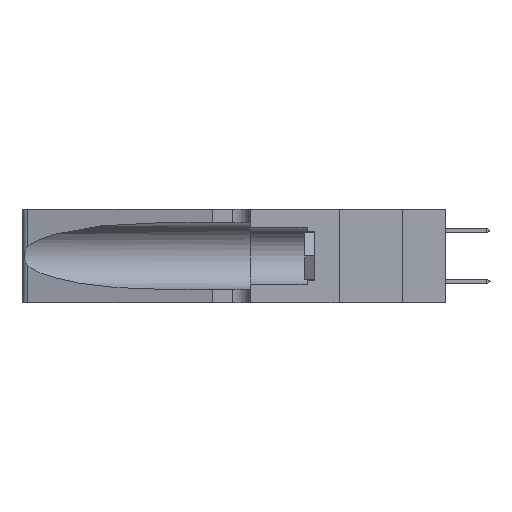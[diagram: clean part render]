
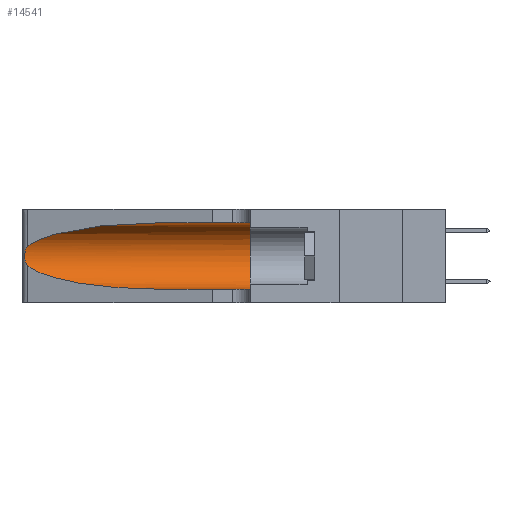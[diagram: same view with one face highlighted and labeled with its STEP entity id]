
A CAD part, left-side view. The second image highlights one B-rep face of the part: STEP entity #14541.
In plain terms, the highlighted cylindrical face has radius 3.308 mm (diameter 6.617 mm), a partial arc.
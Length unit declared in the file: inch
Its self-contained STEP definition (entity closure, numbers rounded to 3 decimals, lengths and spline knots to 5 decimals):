
#385 = ORIENTED_EDGE ( 'NONE', *, *, #40518, .T. ) ;
#543 = VERTEX_POINT ( 'NONE', #14534 ) ;
#595 = VERTEX_POINT ( 'NONE', #36358 ) ;
#2200 = CARTESIAN_POINT ( 'NONE',  ( 0.25639, 1.23186, 0.15144 ) ) ;
#2887 = CARTESIAN_POINT ( 'NONE',  ( 0.1305, 0.35, 0.31525 ) ) ;
#3528 = CARTESIAN_POINT ( 'NONE',  ( 0.25854, 1.2359, 0.20912 ) ) ;
#3661 = CARTESIAN_POINT ( 'NONE',  ( 0.25639, 1.23184, 0.21858 ) ) ;
#4517 = VECTOR ( 'NONE', #16160, 39.37008 ) ;
#4999 = DIRECTION ( 'NONE',  ( 0., -1., 0. ) ) ;
#6022 = VERTEX_POINT ( 'NONE', #2887 ) ;
#6552 = DIRECTION ( 'NONE',  ( 0., 0., 1. ) ) ;
#7584 = EDGE_CURVE ( 'NONE', #6022, #31005, #39950, .T. ) ;
#8187 = CARTESIAN_POINT ( 'NONE',  ( 0.26075, 1.23896, 0.178 ) ) ;
#11516 = LINE ( 'NONE', #19167, #4517 ) ;
#11859 = B_SPLINE_CURVE_WITH_KNOTS ( 'NONE', 3,
 ( #23748, #30055, #3661, #22362, #3528, #25611, #33675, #8187, #33401, #37580, #30331, #2200, #39976, #13443 ),
 .UNSPECIFIED., .F., .F.,
 ( 4, 2, 2, 2, 2, 2, 4 ),
 ( 0., 0.00027, 0.00053, 0.00107, 0.0016, 0.00187, 0.00214 ),
 .UNSPECIFIED. ) ;
#12293 = AXIS2_PLACEMENT_3D ( 'NONE', #34263, #28119, #6552 ) ;
#12368 = FACE_OUTER_BOUND ( 'NONE', #39198, .T. ) ;
#12741 = EDGE_CURVE ( 'NONE', #38311, #595, #11859, .T. ) ;
#13443 = CARTESIAN_POINT ( 'NONE',  ( 0.25487, 1.22718, 0.14631 ) ) ;
#14308 = ORIENTED_EDGE ( 'NONE', *, *, #7584, .F. ) ;
#14534 = CARTESIAN_POINT ( 'NONE',  ( 0.1305, 0.72297, 0.31525 ) ) ;
#14541 = ADVANCED_FACE ( 'NONE', ( #12368 ), #28504, .F. ) ;
#15064 = AXIS2_PLACEMENT_3D ( 'NONE', #24223, #4999, #30131 ) ;
#15164 = EDGE_CURVE ( 'NONE', #543, #6022, #23101, .T. ) ;
#15820 = CARTESIAN_POINT ( 'NONE',  ( 0.25487, 1.22718, 0.22369 ) ) ;
#16160 = DIRECTION ( 'NONE',  ( 0., -1., 0. ) ) ;
#17326 = CARTESIAN_POINT ( 'NONE',  ( 0.18966, 0.96281, 0.05475 ) ) ;
#19167 = CARTESIAN_POINT ( 'NONE',  ( 0.1305, 1.61858, 0.05475 ) ) ;
#19524 = CARTESIAN_POINT ( 'NONE',  ( 0.18966, 0.96281, 0.31525 ) ) ;
#19714 = VECTOR ( 'NONE', #20458, 39.37008 ) ;
#20053 = CARTESIAN_POINT ( 'NONE',  ( 0.1305, 0.72297, 0.05475 ) ) ;
#20215 = ORIENTED_EDGE ( 'NONE', *, *, #15164, .F. ) ;
#20458 = DIRECTION ( 'NONE',  ( 0., -1., 0. ) ) ;
#21467 = CARTESIAN_POINT ( 'NONE',  ( 0.1305, 0.72297, 0.31525 ) ) ;
#21906 = EDGE_CURVE ( 'NONE', #543, #38311, #23351, .T. ) ;
#22362 = CARTESIAN_POINT ( 'NONE',  ( 0.25787, 1.23484, 0.2124 ) ) ;
#22426 = VERTEX_POINT ( 'NONE', #30182 ) ;
#22624 = CARTESIAN_POINT ( 'NONE',  ( 0.25487, 1.22718, 0.22369 ) ) ;
#23101 = LINE ( 'NONE', #26860, #19714 ) ;
#23169 = CARTESIAN_POINT ( 'NONE',  ( 0.2373, 1.15595, 0.08982 ) ) ;
#23351 =( BOUNDED_CURVE ( )  B_SPLINE_CURVE ( 3, ( #21467, #19524, #28958, #22624 ),
 .UNSPECIFIED., .F., .T. ) 
 B_SPLINE_CURVE_WITH_KNOTS ( ( 4, 4 ),
 ( 1.5708, 2.84003 ),
 .UNSPECIFIED. ) 
 CURVE ( )  GEOMETRIC_REPRESENTATION_ITEM ( )  RATIONAL_B_SPLINE_CURVE ( ( 1., 0.87, 0.87, 1. ) ) 
 REPRESENTATION_ITEM ( '' )  );
#23748 = CARTESIAN_POINT ( 'NONE',  ( 0.25487, 1.22718, 0.22369 ) ) ;
#23900 = ORIENTED_EDGE ( 'NONE', *, *, #12741, .T. ) ;
#24223 = CARTESIAN_POINT ( 'NONE',  ( 0.1305, 1.61858, 0.185 ) ) ;
#25611 = CARTESIAN_POINT ( 'NONE',  ( 0.26018, 1.23835, 0.19895 ) ) ;
#26607 = ORIENTED_EDGE ( 'NONE', *, *, #21906, .T. ) ;
#26860 = CARTESIAN_POINT ( 'NONE',  ( 0.1305, 1.61858, 0.31525 ) ) ;
#28119 = DIRECTION ( 'NONE',  ( 0., 1., 0. ) ) ;
#28504 = CYLINDRICAL_SURFACE ( 'NONE', #15064, 0.13025 ) ;
#28857 = CARTESIAN_POINT ( 'NONE',  ( 0.1305, 0.35, 0.05475 ) ) ;
#28958 = CARTESIAN_POINT ( 'NONE',  ( 0.2373, 1.15595, 0.28018 ) ) ;
#29392 = ORIENTED_EDGE ( 'NONE', *, *, #33860, .T. ) ;
#30055 = CARTESIAN_POINT ( 'NONE',  ( 0.25555, 1.22994, 0.2215 ) ) ;
#30131 = DIRECTION ( 'NONE',  ( 0., 0., -1. ) ) ;
#30182 = CARTESIAN_POINT ( 'NONE',  ( 0.1305, 0.72297, 0.05475 ) ) ;
#30331 = CARTESIAN_POINT ( 'NONE',  ( 0.25789, 1.23486, 0.15765 ) ) ;
#31005 = VERTEX_POINT ( 'NONE', #28857 ) ;
#33401 = CARTESIAN_POINT ( 'NONE',  ( 0.26017, 1.23833, 0.17102 ) ) ;
#33675 = CARTESIAN_POINT ( 'NONE',  ( 0.26075, 1.23896, 0.19203 ) ) ;
#33860 = EDGE_CURVE ( 'NONE', #22426, #31005, #11516, .T. ) ;
#34263 = CARTESIAN_POINT ( 'NONE',  ( 0.1305, 0.35, 0.185 ) ) ;
#36358 = CARTESIAN_POINT ( 'NONE',  ( 0.25487, 1.22718, 0.14631 ) ) ;
#37580 = CARTESIAN_POINT ( 'NONE',  ( 0.25856, 1.23593, 0.16098 ) ) ;
#38311 = VERTEX_POINT ( 'NONE', #15820 ) ;
#38764 = CARTESIAN_POINT ( 'NONE',  ( 0.25487, 1.22718, 0.14631 ) ) ;
#39198 = EDGE_LOOP ( 'NONE', ( #26607, #23900, #385, #29392, #14308, #20215 ) ) ;
#39694 =( BOUNDED_CURVE ( )  B_SPLINE_CURVE ( 3, ( #38764, #23169, #17326, #20053 ),
 .UNSPECIFIED., .F., .F. ) 
 B_SPLINE_CURVE_WITH_KNOTS ( ( 4, 4 ),
 ( 3.44316, 4.71239 ),
 .UNSPECIFIED. ) 
 CURVE ( )  GEOMETRIC_REPRESENTATION_ITEM ( )  RATIONAL_B_SPLINE_CURVE ( ( 1., 0.87, 0.87, 1. ) ) 
 REPRESENTATION_ITEM ( '' )  );
#39950 = CIRCLE ( 'NONE', #12293, 0.13025 ) ;
#39976 = CARTESIAN_POINT ( 'NONE',  ( 0.25555, 1.22993, 0.14849 ) ) ;
#40518 = EDGE_CURVE ( 'NONE', #595, #22426, #39694, .T. ) ;
